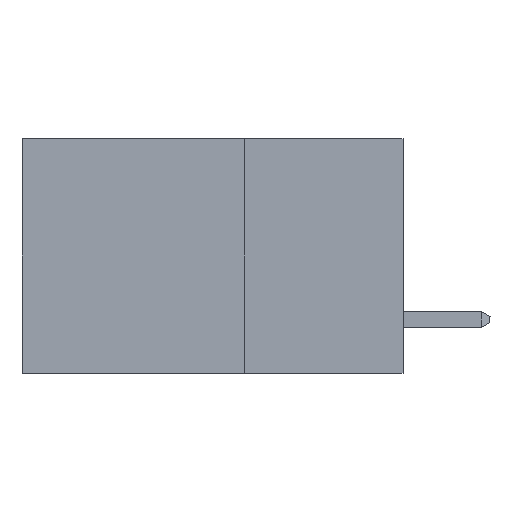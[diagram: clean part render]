
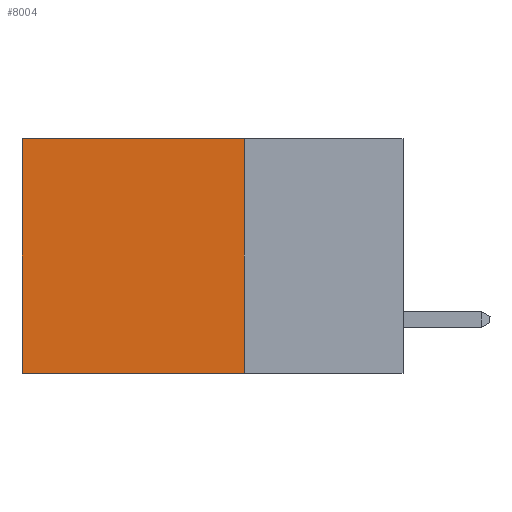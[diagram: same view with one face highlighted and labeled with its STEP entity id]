
A CAD part, left-side view. The second image highlights one B-rep face of the part: STEP entity #8004.
In plain terms, the highlighted planar face has unit normal (-1, 0, 0).
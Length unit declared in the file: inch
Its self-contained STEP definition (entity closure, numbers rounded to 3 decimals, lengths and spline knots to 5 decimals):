
#110 = CARTESIAN_POINT ( 'NONE',  ( 0.2875, 0.25, 0. ) ) ;
#514 = DIRECTION ( 'NONE',  ( 0., 1., 0. ) ) ;
#1126 = EDGE_CURVE ( 'NONE', #29457, #13569, #10858, .T. ) ;
#2093 = VECTOR ( 'NONE', #514, 39.37008 ) ;
#2821 = DIRECTION ( 'NONE',  ( 0., 0., -1. ) ) ;
#3155 = ORIENTED_EDGE ( 'NONE', *, *, #16267, .T. ) ;
#4024 = VERTEX_POINT ( 'NONE', #26713 ) ;
#6271 = ORIENTED_EDGE ( 'NONE', *, *, #15840, .F. ) ;
#7746 = AXIS2_PLACEMENT_3D ( 'NONE', #20297, #32468, #38487 ) ;
#8004 = ADVANCED_FACE ( 'NONE', ( #21833 ), #14023, .F. ) ;
#8481 = ORIENTED_EDGE ( 'NONE', *, *, #1126, .F. ) ;
#9173 = DIRECTION ( 'NONE',  ( 0., 0., -1. ) ) ;
#10200 = LINE ( 'NONE', #110, #2093 ) ;
#10858 = LINE ( 'NONE', #27065, #11834 ) ;
#11353 = LINE ( 'NONE', #13632, #33386 ) ;
#11834 = VECTOR ( 'NONE', #9173, 39.37008 ) ;
#13569 = VERTEX_POINT ( 'NONE', #13684 ) ;
#13632 = CARTESIAN_POINT ( 'NONE',  ( 0.2875, 0.25, -0.37 ) ) ;
#13684 = CARTESIAN_POINT ( 'NONE',  ( 0.2875, 0.25, -0.37 ) ) ;
#14023 = PLANE ( 'NONE',  #7746 ) ;
#15026 = CARTESIAN_POINT ( 'NONE',  ( 0.2875, 0.6, 0. ) ) ;
#15098 = VECTOR ( 'NONE', #2821, 39.37008 ) ;
#15840 = EDGE_CURVE ( 'NONE', #13569, #4024, #11353, .T. ) ;
#16267 = EDGE_CURVE ( 'NONE', #29457, #22121, #10200, .T. ) ;
#20297 = CARTESIAN_POINT ( 'NONE',  ( 0.2875, 0.25, 0. ) ) ;
#20649 = CARTESIAN_POINT ( 'NONE',  ( 0.2875, 0.25, 0. ) ) ;
#20995 = CARTESIAN_POINT ( 'NONE',  ( 0.2875, 0.6, 0. ) ) ;
#21833 = FACE_OUTER_BOUND ( 'NONE', #32385, .T. ) ;
#22121 = VERTEX_POINT ( 'NONE', #15026 ) ;
#22842 = DIRECTION ( 'NONE',  ( 0., 1., 0. ) ) ;
#26713 = CARTESIAN_POINT ( 'NONE',  ( 0.2875, 0.6, -0.37 ) ) ;
#27065 = CARTESIAN_POINT ( 'NONE',  ( 0.2875, 0.25, 0. ) ) ;
#29457 = VERTEX_POINT ( 'NONE', #20649 ) ;
#30410 = LINE ( 'NONE', #20995, #15098 ) ;
#32385 = EDGE_LOOP ( 'NONE', ( #33457, #6271, #8481, #3155 ) ) ;
#32468 = DIRECTION ( 'NONE',  ( 1., 0., 0. ) ) ;
#33386 = VECTOR ( 'NONE', #22842, 39.37008 ) ;
#33457 = ORIENTED_EDGE ( 'NONE', *, *, #37946, .T. ) ;
#37946 = EDGE_CURVE ( 'NONE', #22121, #4024, #30410, .T. ) ;
#38487 = DIRECTION ( 'NONE',  ( 0., 0., -1. ) ) ;
